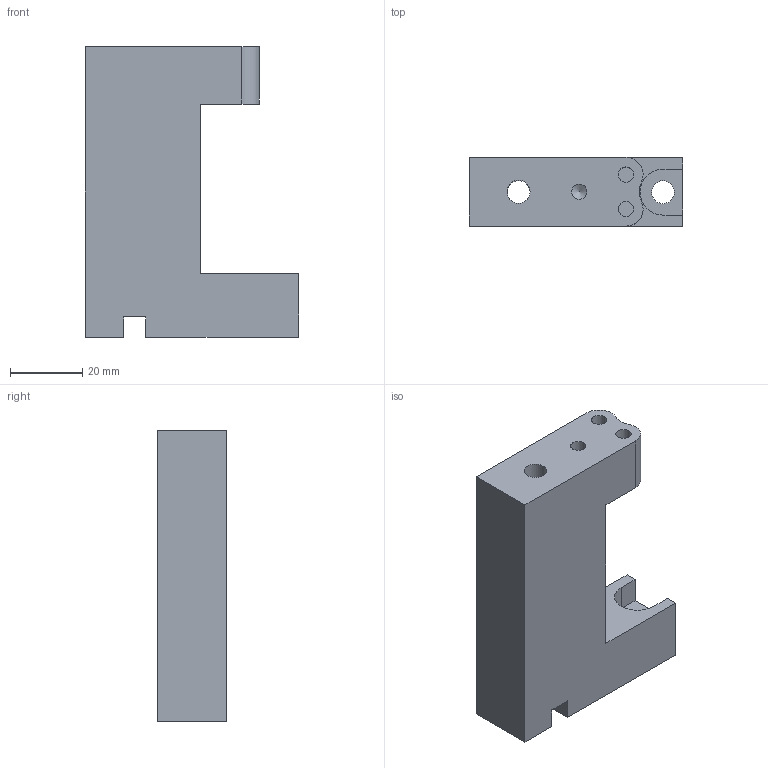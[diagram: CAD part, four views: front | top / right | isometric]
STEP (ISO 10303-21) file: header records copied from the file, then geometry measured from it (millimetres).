
FILE_DESCRIPTION(/* description */ (''),/* implementation_level */ '2;1');
FILE_NAME(/* name */ 'CLAMP-01 - Body revA.step',/* time_stamp */ '2021-11-08T14:09:15-06:00',/* author */ (''),/* organization */ (''),/* preprocessor_version */ 'ST-DEVELOPER v18.1',/* originating_system */ 'Autodesk Translation Framework v10.10.0.1391',/* authorisation */ '');
FILE_SCHEMA (('AUTOMOTIVE_DESIGN { 1 0 10303 214 3 1 1 }'));
Length unit declared in the file: inch
Products named in the file (1): CLAMP-01 - Body
Bounding box: 59.05 x 19.05 x 80.52 mm (x, y, z)
Volume: 57710 mm3; surface area: 14773.2 mm2
Topology: 1 solids, 1 shells, 29 faces, 83 edges, 55 vertices
Faces by surface type: plane 19, cylinder 9, cone 1
Full cylindrical faces by diameter (mm): 4.234 x3, 6.35 x2
Entity records: 1004 total; most frequent: CARTESIAN_POINT 167, ORIENTED_EDGE 164, DIRECTION 164, EDGE_CURVE 82, LINE 60, VECTOR 60, VERTEX_POINT 55, AXIS2_PLACEMENT_3D 52
